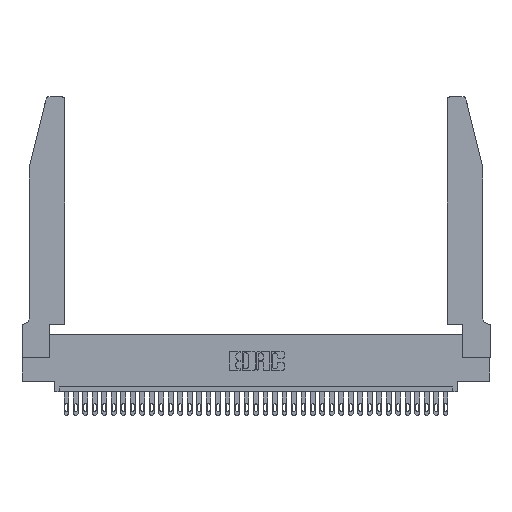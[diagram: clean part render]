
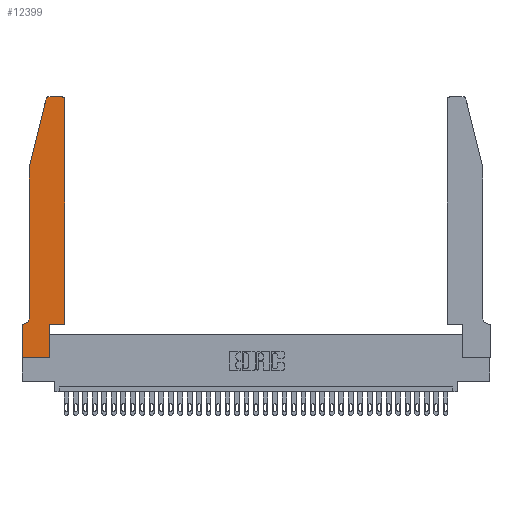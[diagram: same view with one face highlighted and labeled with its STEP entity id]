
A CAD part, top view. The second image highlights one B-rep face of the part: STEP entity #12399.
In plain terms, the highlighted planar face has unit normal (0, 0, 1).
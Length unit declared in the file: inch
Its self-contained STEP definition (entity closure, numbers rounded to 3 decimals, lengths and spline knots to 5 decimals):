
#196 = LINE ( 'NONE', #31426, #13179 ) ;
#202 = ORIENTED_EDGE ( 'NONE', *, *, #34285, .T. ) ;
#714 = CARTESIAN_POINT ( 'NONE',  ( 0.4505, 0.35, 0.37 ) ) ;
#1165 = CARTESIAN_POINT ( 'NONE',  ( 0.0755, 2., 0.37 ) ) ;
#1312 = CARTESIAN_POINT ( 'NONE',  ( 0., 0.35, 0.37 ) ) ;
#1612 = CARTESIAN_POINT ( 'NONE',  ( 0.4205, 2.72, 0.37 ) ) ;
#2493 = VECTOR ( 'NONE', #23947, 39.37008 ) ;
#3365 = ORIENTED_EDGE ( 'NONE', *, *, #21606, .T. ) ;
#3573 = VERTEX_POINT ( 'NONE', #9159 ) ;
#3648 = DIRECTION ( 'NONE',  ( -1., 0., 0. ) ) ;
#3926 = DIRECTION ( 'NONE',  ( 0., 0., -1. ) ) ;
#3980 = ORIENTED_EDGE ( 'NONE', *, *, #17271, .T. ) ;
#4993 = CARTESIAN_POINT ( 'NONE',  ( 0.284, 2.75, 0.37 ) ) ;
#5234 = LINE ( 'NONE', #28068, #26422 ) ;
#5696 = VERTEX_POINT ( 'NONE', #19122 ) ;
#5765 = CARTESIAN_POINT ( 'NONE',  ( 0.0755, 0.35, 0.37 ) ) ;
#6269 = LINE ( 'NONE', #1165, #34871 ) ;
#6480 = DIRECTION ( 'NONE',  ( 0., 0., 1. ) ) ;
#6856 = CARTESIAN_POINT ( 'NONE',  ( 0., 0.35, 0.37 ) ) ;
#7844 = VERTEX_POINT ( 'NONE', #9738 ) ;
#7851 = AXIS2_PLACEMENT_3D ( 'NONE', #1612, #23760, #9465 ) ;
#7953 = AXIS2_PLACEMENT_3D ( 'NONE', #14208, #28247, #28627 ) ;
#8289 = VECTOR ( 'NONE', #32481, 39.37008 ) ;
#9159 = CARTESIAN_POINT ( 'NONE',  ( 0., 0., 0.37 ) ) ;
#9193 = EDGE_CURVE ( 'NONE', #14966, #13347, #24710, .T. ) ;
#9465 = DIRECTION ( 'NONE',  ( 1., 0., 0. ) ) ;
#9738 = CARTESIAN_POINT ( 'NONE',  ( 0.0755, 0.42, 0.37 ) ) ;
#11688 = ORIENTED_EDGE ( 'NONE', *, *, #27662, .T. ) ;
#12399 = ADVANCED_FACE ( 'NONE', ( #22303 ), #23075, .T. ) ;
#13170 = ORIENTED_EDGE ( 'NONE', *, *, #14840, .T. ) ;
#13179 = VECTOR ( 'NONE', #26137, 39.37008 ) ;
#13347 = VERTEX_POINT ( 'NONE', #4993 ) ;
#14208 = CARTESIAN_POINT ( 'NONE',  ( 0.284, 2.72, 0.37 ) ) ;
#14472 = CIRCLE ( 'NONE', #7953, 0.03 ) ;
#14840 = EDGE_CURVE ( 'NONE', #5696, #15871, #17624, .T. ) ;
#14859 = DIRECTION ( 'NONE',  ( 0., 1., 0. ) ) ;
#14966 = VERTEX_POINT ( 'NONE', #34704 ) ;
#15147 = AXIS2_PLACEMENT_3D ( 'NONE', #17563, #3926, #3648 ) ;
#15804 = EDGE_CURVE ( 'NONE', #13347, #22419, #14472, .T. ) ;
#15871 = VERTEX_POINT ( 'NONE', #22536 ) ;
#15924 = CARTESIAN_POINT ( 'NONE',  ( 0.2605, 2.75, 0.37 ) ) ;
#15999 = EDGE_CURVE ( 'NONE', #23745, #7844, #6269, .T. ) ;
#17271 = EDGE_CURVE ( 'NONE', #18870, #3573, #196, .T. ) ;
#17563 = CARTESIAN_POINT ( 'NONE',  ( 0.0055, 0.42, 0.37 ) ) ;
#17624 = LINE ( 'NONE', #714, #35809 ) ;
#18415 = ORIENTED_EDGE ( 'NONE', *, *, #15999, .T. ) ;
#18870 = VERTEX_POINT ( 'NONE', #6856 ) ;
#19122 = CARTESIAN_POINT ( 'NONE',  ( 0.4505, 0.35, 0.37 ) ) ;
#19254 = ORIENTED_EDGE ( 'NONE', *, *, #24997, .T. ) ;
#19379 = VERTEX_POINT ( 'NONE', #34643 ) ;
#20609 = CARTESIAN_POINT ( 'NONE',  ( 0.25487, 2.72718, 0.37 ) ) ;
#20679 = DIRECTION ( 'NONE',  ( 1., 0., 0. ) ) ;
#20875 = CARTESIAN_POINT ( 'NONE',  ( 0.0755, 2., 0.37 ) ) ;
#21000 = VECTOR ( 'NONE', #23652, 39.37008 ) ;
#21459 = ORIENTED_EDGE ( 'NONE', *, *, #33171, .T. ) ;
#21606 = EDGE_CURVE ( 'NONE', #15871, #14966, #30543, .T. ) ;
#21635 = VECTOR ( 'NONE', #28340, 39.37008 ) ;
#21775 = ORIENTED_EDGE ( 'NONE', *, *, #25937, .T. ) ;
#22303 = FACE_OUTER_BOUND ( 'NONE', #30534, .T. ) ;
#22419 = VERTEX_POINT ( 'NONE', #20609 ) ;
#22505 = LINE ( 'NONE', #23943, #8289 ) ;
#22536 = CARTESIAN_POINT ( 'NONE',  ( 0.4505, 2.72, 0.37 ) ) ;
#22771 = DIRECTION ( 'NONE',  ( 0., -1., 0. ) ) ;
#23075 = PLANE ( 'NONE',  #24509 ) ;
#23181 = DIRECTION ( 'NONE',  ( 1., 0., 0. ) ) ;
#23457 = CARTESIAN_POINT ( 'NONE',  ( 0.4505, 0.35, 0.37 ) ) ;
#23652 = DIRECTION ( 'NONE',  ( -0.239, -0.971, 0. ) ) ;
#23745 = VERTEX_POINT ( 'NONE', #20875 ) ;
#23760 = DIRECTION ( 'NONE',  ( 0., 0., 1. ) ) ;
#23943 = CARTESIAN_POINT ( 'NONE',  ( 0.2865, 0.35, 0.37 ) ) ;
#23947 = DIRECTION ( 'NONE',  ( 1., 0., 0. ) ) ;
#24087 = CIRCLE ( 'NONE', #15147, 0.07 ) ;
#24509 = AXIS2_PLACEMENT_3D ( 'NONE', #1312, #6480, #20679 ) ;
#24710 = LINE ( 'NONE', #15924, #32488 ) ;
#24997 = EDGE_CURVE ( 'NONE', #25546, #32218, #22505, .T. ) ;
#25546 = VERTEX_POINT ( 'NONE', #32257 ) ;
#25937 = EDGE_CURVE ( 'NONE', #19379, #18870, #26386, .T. ) ;
#26137 = DIRECTION ( 'NONE',  ( 0., -1., 0. ) ) ;
#26289 = CARTESIAN_POINT ( 'NONE',  ( 0.2865, 0.35, 0.37 ) ) ;
#26386 = LINE ( 'NONE', #5765, #21635 ) ;
#26422 = VECTOR ( 'NONE', #23181, 39.37008 ) ;
#27019 = LINE ( 'NONE', #31591, #21000 ) ;
#27107 = EDGE_CURVE ( 'NONE', #32218, #5696, #27172, .T. ) ;
#27172 = LINE ( 'NONE', #23457, #2493 ) ;
#27432 = ORIENTED_EDGE ( 'NONE', *, *, #27107, .T. ) ;
#27517 = ORIENTED_EDGE ( 'NONE', *, *, #9193, .T. ) ;
#27662 = EDGE_CURVE ( 'NONE', #22419, #23745, #27019, .T. ) ;
#28068 = CARTESIAN_POINT ( 'NONE',  ( 0., 0., 0.37 ) ) ;
#28247 = DIRECTION ( 'NONE',  ( 0., 0., 1. ) ) ;
#28340 = DIRECTION ( 'NONE',  ( -1., 0., 0. ) ) ;
#28627 = DIRECTION ( 'NONE',  ( 1., 0., 0. ) ) ;
#29897 = DIRECTION ( 'NONE',  ( -1., 0., 0. ) ) ;
#30073 = ORIENTED_EDGE ( 'NONE', *, *, #15804, .T. ) ;
#30534 = EDGE_LOOP ( 'NONE', ( #27517, #30073, #11688, #18415, #21459, #21775, #3980, #202, #19254, #27432, #13170, #3365 ) ) ;
#30543 = CIRCLE ( 'NONE', #7851, 0.03 ) ;
#31426 = CARTESIAN_POINT ( 'NONE',  ( 0., 0., 0.37 ) ) ;
#31591 = CARTESIAN_POINT ( 'NONE',  ( 0.0755, 2., 0.37 ) ) ;
#32218 = VERTEX_POINT ( 'NONE', #26289 ) ;
#32257 = CARTESIAN_POINT ( 'NONE',  ( 0.2865, 0., 0.37 ) ) ;
#32481 = DIRECTION ( 'NONE',  ( 0., 1., 0. ) ) ;
#32488 = VECTOR ( 'NONE', #29897, 39.37008 ) ;
#33171 = EDGE_CURVE ( 'NONE', #7844, #19379, #24087, .T. ) ;
#34285 = EDGE_CURVE ( 'NONE', #3573, #25546, #5234, .T. ) ;
#34643 = CARTESIAN_POINT ( 'NONE',  ( 0.0055, 0.35, 0.37 ) ) ;
#34704 = CARTESIAN_POINT ( 'NONE',  ( 0.4205, 2.75, 0.37 ) ) ;
#34871 = VECTOR ( 'NONE', #22771, 39.37008 ) ;
#35809 = VECTOR ( 'NONE', #14859, 39.37008 ) ;
